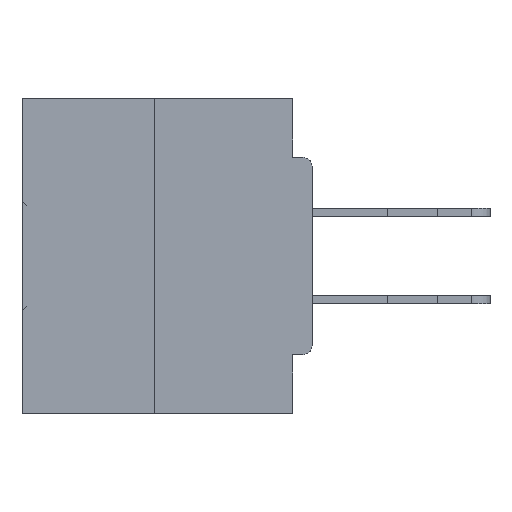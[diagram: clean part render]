
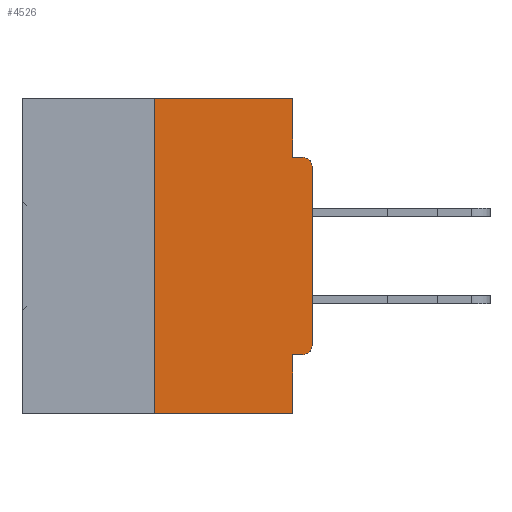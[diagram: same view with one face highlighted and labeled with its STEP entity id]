
A CAD part, left-side view. The second image highlights one B-rep face of the part: STEP entity #4526.
In plain terms, the highlighted planar face has unit normal (-1, 0, 0).
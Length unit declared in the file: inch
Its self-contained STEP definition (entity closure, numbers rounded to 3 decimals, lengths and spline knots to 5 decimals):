
#671 = ORIENTED_EDGE ( 'NONE', *, *, #25155, .F. ) ;
#1111 = VECTOR ( 'NONE', #43612, 39.37008 ) ;
#1727 = LINE ( 'NONE', #8548, #10795 ) ;
#1939 = ORIENTED_EDGE ( 'NONE', *, *, #22318, .T. ) ;
#2089 = CARTESIAN_POINT ( 'NONE',  ( 0., 0.46, -0.5 ) ) ;
#2950 = DIRECTION ( 'NONE',  ( 0., 0., -1. ) ) ;
#3557 = PLANE ( 'NONE',  #16391 ) ;
#4343 = EDGE_CURVE ( 'NONE', #45536, #30804, #27732, .T. ) ;
#4397 = CARTESIAN_POINT ( 'NONE',  ( 0., 0.25, 0. ) ) ;
#4526 = ADVANCED_FACE ( 'NONE', ( #5654 ), #3557, .F. ) ;
#4561 = ORIENTED_EDGE ( 'NONE', *, *, #4343, .F. ) ;
#4959 = EDGE_CURVE ( 'NONE', #31284, #6888, #1727, .T. ) ;
#5254 = CARTESIAN_POINT ( 'NONE',  ( 0., 0.031, -0.4065 ) ) ;
#5648 = VECTOR ( 'NONE', #17469, 39.37008 ) ;
#5654 = FACE_OUTER_BOUND ( 'NONE', #16899, .T. ) ;
#6888 = VERTEX_POINT ( 'NONE', #5254 ) ;
#8225 = DIRECTION ( 'NONE',  ( 0., -1., 0. ) ) ;
#8374 = CIRCLE ( 'NONE', #27661, 0.015 ) ;
#8548 = CARTESIAN_POINT ( 'NONE',  ( 0., 0., -0.4065 ) ) ;
#9002 = EDGE_CURVE ( 'NONE', #37423, #45393, #40108, .T. ) ;
#10169 = VECTOR ( 'NONE', #45293, 39.37008 ) ;
#10795 = VECTOR ( 'NONE', #37755, 39.37008 ) ;
#11238 = CARTESIAN_POINT ( 'NONE',  ( 0., 0.031, -0.5 ) ) ;
#12059 = VERTEX_POINT ( 'NONE', #38334 ) ;
#12263 = DIRECTION ( 'NONE',  ( -1., 0., 0. ) ) ;
#12397 = LINE ( 'NONE', #25804, #37271 ) ;
#13153 = DIRECTION ( 'NONE',  ( -1., 0., 0. ) ) ;
#13388 = CARTESIAN_POINT ( 'NONE',  ( 0., 0.031, -0.5 ) ) ;
#14153 = DIRECTION ( 'NONE',  ( 1., 0., 0. ) ) ;
#14808 = ORIENTED_EDGE ( 'NONE', *, *, #9002, .F. ) ;
#16391 = AXIS2_PLACEMENT_3D ( 'NONE', #46316, #14153, #2950 ) ;
#16606 = CIRCLE ( 'NONE', #46795, 0.015 ) ;
#16899 = EDGE_LOOP ( 'NONE', ( #45277, #4561, #27080, #671, #37660, #40576, #35361, #1939, #42374, #14808 ) ) ;
#16943 = CARTESIAN_POINT ( 'NONE',  ( 0., 0.25, -0.5 ) ) ;
#17469 = DIRECTION ( 'NONE',  ( 0., 0., -1. ) ) ;
#17705 = VERTEX_POINT ( 'NONE', #40082 ) ;
#19158 = EDGE_CURVE ( 'NONE', #45536, #30015, #27689, .T. ) ;
#19371 = DIRECTION ( 'NONE',  ( 0., 0., -1. ) ) ;
#19705 = EDGE_CURVE ( 'NONE', #45393, #21925, #41777, .T. ) ;
#21925 = VERTEX_POINT ( 'NONE', #37223 ) ;
#22318 = EDGE_CURVE ( 'NONE', #17705, #21925, #16606, .T. ) ;
#22779 = DIRECTION ( 'NONE',  ( 0., 0., 1. ) ) ;
#24479 = VECTOR ( 'NONE', #30386, 39.37008 ) ;
#25155 = EDGE_CURVE ( 'NONE', #6888, #30015, #36747, .T. ) ;
#25804 = CARTESIAN_POINT ( 'NONE',  ( 0., 0.46, 0. ) ) ;
#26609 = VECTOR ( 'NONE', #22779, 39.37008 ) ;
#27080 = ORIENTED_EDGE ( 'NONE', *, *, #19158, .T. ) ;
#27661 = AXIS2_PLACEMENT_3D ( 'NONE', #30430, #12263, #19371 ) ;
#27689 = LINE ( 'NONE', #2089, #10169 ) ;
#27732 = LINE ( 'NONE', #4397, #26609 ) ;
#28263 = CARTESIAN_POINT ( 'NONE',  ( 0., 0.25, 0. ) ) ;
#29647 = EDGE_CURVE ( 'NONE', #12059, #17705, #36320, .T. ) ;
#29853 = CARTESIAN_POINT ( 'NONE',  ( 0., 0., -0.0935 ) ) ;
#30015 = VERTEX_POINT ( 'NONE', #11238 ) ;
#30386 = DIRECTION ( 'NONE',  ( 0., 0., 1. ) ) ;
#30430 = CARTESIAN_POINT ( 'NONE',  ( 0., 0.015, -0.3915 ) ) ;
#30713 = DIRECTION ( 'NONE',  ( 0., 0., -1. ) ) ;
#30804 = VERTEX_POINT ( 'NONE', #28263 ) ;
#31165 = CARTESIAN_POINT ( 'NONE',  ( 0., 0.015, -0.1085 ) ) ;
#31284 = VERTEX_POINT ( 'NONE', #34229 ) ;
#34178 = CARTESIAN_POINT ( 'NONE',  ( 0., 0., 0. ) ) ;
#34229 = CARTESIAN_POINT ( 'NONE',  ( 0., 0.015, -0.4065 ) ) ;
#35361 = ORIENTED_EDGE ( 'NONE', *, *, #29647, .T. ) ;
#36320 = LINE ( 'NONE', #34178, #24479 ) ;
#36574 = EDGE_CURVE ( 'NONE', #31284, #12059, #8374, .T. ) ;
#36747 = LINE ( 'NONE', #13388, #5648 ) ;
#37223 = CARTESIAN_POINT ( 'NONE',  ( 0., 0.015, -0.0935 ) ) ;
#37271 = VECTOR ( 'NONE', #45274, 39.37008 ) ;
#37423 = VERTEX_POINT ( 'NONE', #42851 ) ;
#37498 = CARTESIAN_POINT ( 'NONE',  ( 0., 0.031, -0.0935 ) ) ;
#37660 = ORIENTED_EDGE ( 'NONE', *, *, #4959, .F. ) ;
#37755 = DIRECTION ( 'NONE',  ( 0., 1., 0. ) ) ;
#38334 = CARTESIAN_POINT ( 'NONE',  ( 0., 0., -0.3915 ) ) ;
#39931 = CARTESIAN_POINT ( 'NONE',  ( 0., 0.031, 0. ) ) ;
#40071 = VECTOR ( 'NONE', #8225, 39.37008 ) ;
#40082 = CARTESIAN_POINT ( 'NONE',  ( 0., 0., -0.1085 ) ) ;
#40108 = LINE ( 'NONE', #39931, #1111 ) ;
#40576 = ORIENTED_EDGE ( 'NONE', *, *, #36574, .T. ) ;
#41026 = EDGE_CURVE ( 'NONE', #30804, #37423, #12397, .T. ) ;
#41777 = LINE ( 'NONE', #29853, #40071 ) ;
#42374 = ORIENTED_EDGE ( 'NONE', *, *, #19705, .F. ) ;
#42851 = CARTESIAN_POINT ( 'NONE',  ( 0., 0.031, 0. ) ) ;
#43612 = DIRECTION ( 'NONE',  ( 0., 0., -1. ) ) ;
#45274 = DIRECTION ( 'NONE',  ( 0., -1., 0. ) ) ;
#45277 = ORIENTED_EDGE ( 'NONE', *, *, #41026, .F. ) ;
#45293 = DIRECTION ( 'NONE',  ( 0., -1., 0. ) ) ;
#45393 = VERTEX_POINT ( 'NONE', #37498 ) ;
#45536 = VERTEX_POINT ( 'NONE', #16943 ) ;
#46316 = CARTESIAN_POINT ( 'NONE',  ( 0., 0.46, 0. ) ) ;
#46795 = AXIS2_PLACEMENT_3D ( 'NONE', #31165, #13153, #30713 ) ;
